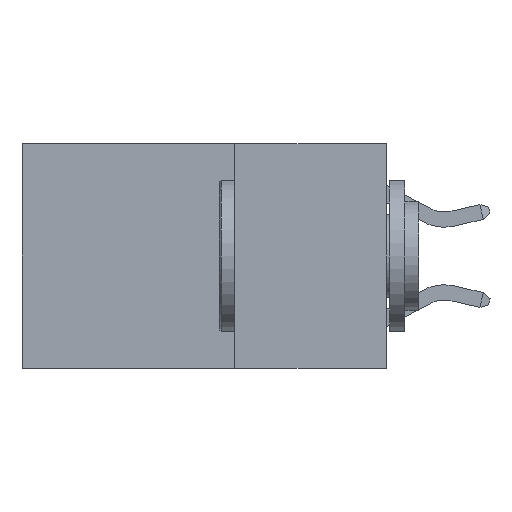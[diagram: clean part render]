
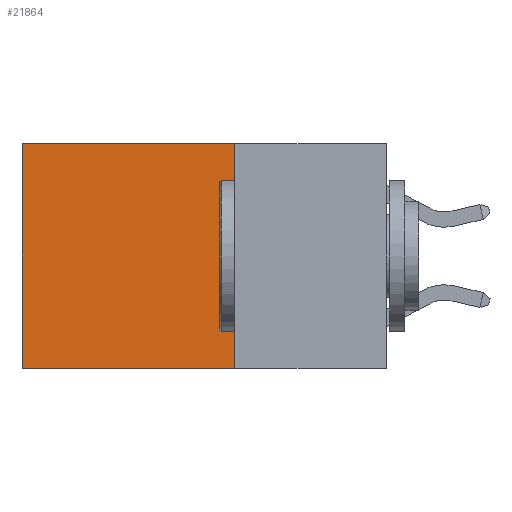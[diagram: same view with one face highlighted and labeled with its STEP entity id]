
A CAD part, left-side view. The second image highlights one B-rep face of the part: STEP entity #21864.
In plain terms, the highlighted planar face has unit normal (-1, 0, 0).
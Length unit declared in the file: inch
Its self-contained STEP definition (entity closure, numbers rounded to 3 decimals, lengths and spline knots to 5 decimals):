
#231 = EDGE_CURVE ( 'NONE', #16905, #28972, #17489, .T. ) ;
#1481 = VECTOR ( 'NONE', #27624, 39.37008 ) ;
#2919 = EDGE_LOOP ( 'NONE', ( #17575, #27723, #9223, #6017 ) ) ;
#4973 = EDGE_CURVE ( 'NONE', #24867, #5254, #9553, .T. ) ;
#5254 = VERTEX_POINT ( 'NONE', #28048 ) ;
#6017 = ORIENTED_EDGE ( 'NONE', *, *, #28917, .T. ) ;
#6208 = CARTESIAN_POINT ( 'NONE',  ( 0.2625, 0.6, -0.37 ) ) ;
#8926 = DIRECTION ( 'NONE',  ( 1., 0., 0. ) ) ;
#9223 = ORIENTED_EDGE ( 'NONE', *, *, #4973, .F. ) ;
#9553 = LINE ( 'NONE', #14468, #15903 ) ;
#10815 = CARTESIAN_POINT ( 'NONE',  ( 0.2625, 0.6, 0. ) ) ;
#14468 = CARTESIAN_POINT ( 'NONE',  ( 0.2625, 0.25, 0. ) ) ;
#14578 = VECTOR ( 'NONE', #17646, 39.37008 ) ;
#15903 = VECTOR ( 'NONE', #26364, 39.37008 ) ;
#16221 = AXIS2_PLACEMENT_3D ( 'NONE', #20837, #8926, #20996 ) ;
#16905 = VERTEX_POINT ( 'NONE', #26824 ) ;
#17312 = DIRECTION ( 'NONE',  ( 0., 1., 0. ) ) ;
#17489 = LINE ( 'NONE', #10815, #1481 ) ;
#17575 = ORIENTED_EDGE ( 'NONE', *, *, #231, .T. ) ;
#17646 = DIRECTION ( 'NONE',  ( 0., 1., 0. ) ) ;
#18296 = VECTOR ( 'NONE', #17312, 39.37008 ) ;
#19672 = LINE ( 'NONE', #29356, #18296 ) ;
#19673 = CARTESIAN_POINT ( 'NONE',  ( 0.2625, 0.25, 0. ) ) ;
#20179 = CARTESIAN_POINT ( 'NONE',  ( 0.2625, 0.25, 0. ) ) ;
#20822 = EDGE_CURVE ( 'NONE', #5254, #28972, #19672, .T. ) ;
#20837 = CARTESIAN_POINT ( 'NONE',  ( 0.2625, 0.25, 0. ) ) ;
#20996 = DIRECTION ( 'NONE',  ( 0., 0., -1. ) ) ;
#21864 = ADVANCED_FACE ( 'NONE', ( #30660 ), #22323, .F. ) ;
#22258 = LINE ( 'NONE', #20179, #14578 ) ;
#22323 = PLANE ( 'NONE',  #16221 ) ;
#24867 = VERTEX_POINT ( 'NONE', #19673 ) ;
#26364 = DIRECTION ( 'NONE',  ( 0., 0., -1. ) ) ;
#26824 = CARTESIAN_POINT ( 'NONE',  ( 0.2625, 0.6, 0. ) ) ;
#27624 = DIRECTION ( 'NONE',  ( 0., 0., -1. ) ) ;
#27723 = ORIENTED_EDGE ( 'NONE', *, *, #20822, .F. ) ;
#28048 = CARTESIAN_POINT ( 'NONE',  ( 0.2625, 0.25, -0.37 ) ) ;
#28917 = EDGE_CURVE ( 'NONE', #24867, #16905, #22258, .T. ) ;
#28972 = VERTEX_POINT ( 'NONE', #6208 ) ;
#29356 = CARTESIAN_POINT ( 'NONE',  ( 0.2625, 0.25, -0.37 ) ) ;
#30660 = FACE_OUTER_BOUND ( 'NONE', #2919, .T. ) ;
